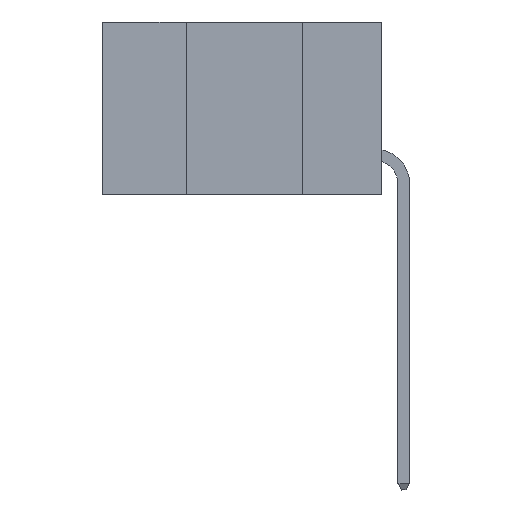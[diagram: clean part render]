
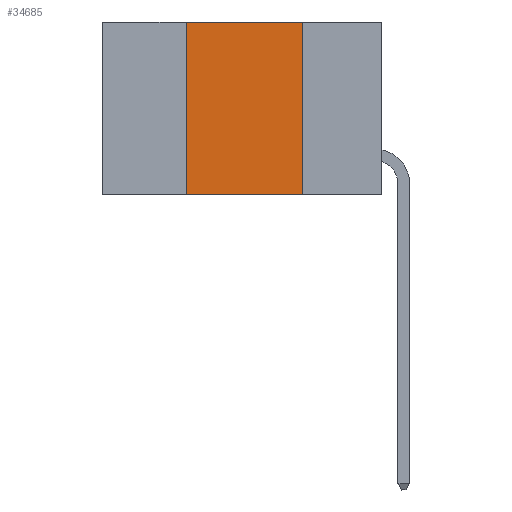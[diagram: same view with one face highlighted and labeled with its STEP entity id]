
A CAD part, left-side view. The second image highlights one B-rep face of the part: STEP entity #34685.
In plain terms, the highlighted planar face has unit normal (-1, 0, 0).
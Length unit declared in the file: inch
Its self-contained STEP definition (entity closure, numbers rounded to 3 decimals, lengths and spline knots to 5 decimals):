
#2814 = LINE ( 'NONE', #48396, #8243 ) ;
#5856 = CARTESIAN_POINT ( 'NONE',  ( 0., 0.42, 0. ) ) ;
#8243 = VECTOR ( 'NONE', #40068, 39.37008 ) ;
#9357 = VERTEX_POINT ( 'NONE', #14355 ) ;
#9658 = CARTESIAN_POINT ( 'NONE',  ( 0., 0.17, -0.37 ) ) ;
#11748 = EDGE_CURVE ( 'NONE', #12387, #31693, #43662, .T. ) ;
#12387 = VERTEX_POINT ( 'NONE', #41586 ) ;
#12681 = FACE_OUTER_BOUND ( 'NONE', #35477, .T. ) ;
#12813 = DIRECTION ( 'NONE',  ( 0., -1., 0. ) ) ;
#13072 = CARTESIAN_POINT ( 'NONE',  ( 0., 0.6, 0. ) ) ;
#13675 = DIRECTION ( 'NONE',  ( 0., 0., 1. ) ) ;
#14355 = CARTESIAN_POINT ( 'NONE',  ( 0., 0.42, -0.37 ) ) ;
#14912 = VERTEX_POINT ( 'NONE', #19405 ) ;
#16453 = ORIENTED_EDGE ( 'NONE', *, *, #29898, .F. ) ;
#19405 = CARTESIAN_POINT ( 'NONE',  ( 0., 0.42, 0. ) ) ;
#20478 = ORIENTED_EDGE ( 'NONE', *, *, #11748, .F. ) ;
#21053 = DIRECTION ( 'NONE',  ( 0., 0., -1. ) ) ;
#21212 = CARTESIAN_POINT ( 'NONE',  ( 0., 0.17, 0. ) ) ;
#25456 = AXIS2_PLACEMENT_3D ( 'NONE', #13072, #32238, #31915 ) ;
#28173 = ORIENTED_EDGE ( 'NONE', *, *, #31649, .T. ) ;
#28285 = EDGE_CURVE ( 'NONE', #14912, #12387, #31096, .T. ) ;
#29898 = EDGE_CURVE ( 'NONE', #9357, #14912, #30341, .T. ) ;
#30341 = LINE ( 'NONE', #5856, #41932 ) ;
#31096 = LINE ( 'NONE', #39671, #32929 ) ;
#31649 = EDGE_CURVE ( 'NONE', #9357, #31693, #2814, .T. ) ;
#31693 = VERTEX_POINT ( 'NONE', #9658 ) ;
#31915 = DIRECTION ( 'NONE',  ( 0., 0., -1. ) ) ;
#32238 = DIRECTION ( 'NONE',  ( 1., 0., 0. ) ) ;
#32929 = VECTOR ( 'NONE', #12813, 39.37008 ) ;
#34685 = ADVANCED_FACE ( 'NONE', ( #12681 ), #46897, .F. ) ;
#35477 = EDGE_LOOP ( 'NONE', ( #20478, #38980, #16453, #28173 ) ) ;
#38980 = ORIENTED_EDGE ( 'NONE', *, *, #28285, .F. ) ;
#39671 = CARTESIAN_POINT ( 'NONE',  ( 0., 0.6, 0. ) ) ;
#40068 = DIRECTION ( 'NONE',  ( 0., -1., 0. ) ) ;
#41279 = VECTOR ( 'NONE', #21053, 39.37008 ) ;
#41586 = CARTESIAN_POINT ( 'NONE',  ( 0., 0.17, 0. ) ) ;
#41932 = VECTOR ( 'NONE', #13675, 39.37008 ) ;
#43662 = LINE ( 'NONE', #21212, #41279 ) ;
#46897 = PLANE ( 'NONE',  #25456 ) ;
#48396 = CARTESIAN_POINT ( 'NONE',  ( 0., 0.6, -0.37 ) ) ;
